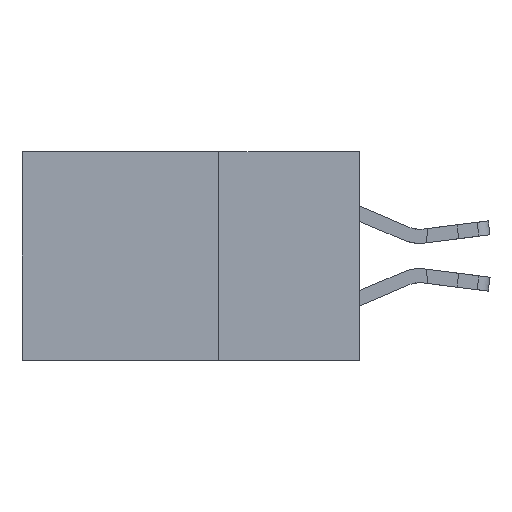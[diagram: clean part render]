
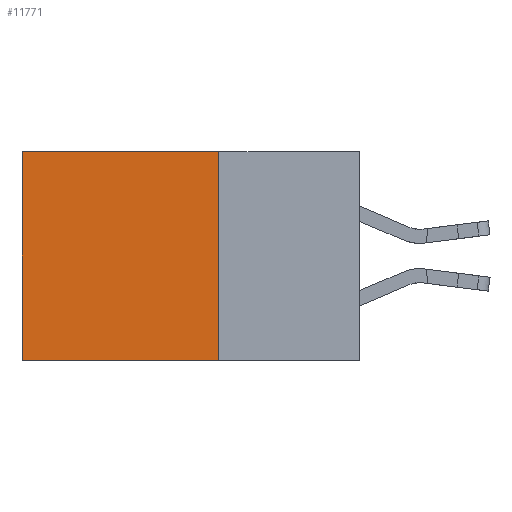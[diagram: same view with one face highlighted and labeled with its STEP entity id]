
A CAD part, left-side view. The second image highlights one B-rep face of the part: STEP entity #11771.
In plain terms, the highlighted planar face has unit normal (-1, 0, 0).
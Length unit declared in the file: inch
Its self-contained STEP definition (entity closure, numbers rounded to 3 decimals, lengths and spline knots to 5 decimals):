
#40 = EDGE_CURVE ( 'NONE', #6525, #1694, #21923, .T. ) ;
#1694 = VERTEX_POINT ( 'NONE', #3701 ) ;
#2074 = VECTOR ( 'NONE', #22208, 39.37008 ) ;
#2262 = CARTESIAN_POINT ( 'NONE',  ( 0.2875, 0.6, -0.37 ) ) ;
#2395 = DIRECTION ( 'NONE',  ( 0., 0., -1. ) ) ;
#2491 = CARTESIAN_POINT ( 'NONE',  ( 0.2875, 0.6, 0. ) ) ;
#3660 = LINE ( 'NONE', #2491, #9148 ) ;
#3701 = CARTESIAN_POINT ( 'NONE',  ( 0.2875, 0.6, 0. ) ) ;
#6525 = VERTEX_POINT ( 'NONE', #13653 ) ;
#6971 = VERTEX_POINT ( 'NONE', #26401 ) ;
#7030 = CARTESIAN_POINT ( 'NONE',  ( 0.2875, 0.25, 0. ) ) ;
#9148 = VECTOR ( 'NONE', #2395, 39.37008 ) ;
#9944 = FACE_OUTER_BOUND ( 'NONE', #11596, .T. ) ;
#10427 = PLANE ( 'NONE',  #12889 ) ;
#10515 = CARTESIAN_POINT ( 'NONE',  ( 0.2875, 0.25, 0. ) ) ;
#10843 = EDGE_CURVE ( 'NONE', #6971, #20252, #19705, .T. ) ;
#11596 = EDGE_LOOP ( 'NONE', ( #14312, #22333, #11752, #15741 ) ) ;
#11752 = ORIENTED_EDGE ( 'NONE', *, *, #15816, .F. ) ;
#11771 = ADVANCED_FACE ( 'NONE', ( #9944 ), #10427, .F. ) ;
#12889 = AXIS2_PLACEMENT_3D ( 'NONE', #10515, #22257, #15390 ) ;
#13653 = CARTESIAN_POINT ( 'NONE',  ( 0.2875, 0.25, 0. ) ) ;
#14096 = EDGE_CURVE ( 'NONE', #1694, #20252, #3660, .T. ) ;
#14312 = ORIENTED_EDGE ( 'NONE', *, *, #14096, .T. ) ;
#14995 = LINE ( 'NONE', #15427, #17056 ) ;
#15390 = DIRECTION ( 'NONE',  ( 0., 0., -1. ) ) ;
#15427 = CARTESIAN_POINT ( 'NONE',  ( 0.2875, 0.25, 0. ) ) ;
#15741 = ORIENTED_EDGE ( 'NONE', *, *, #40, .T. ) ;
#15816 = EDGE_CURVE ( 'NONE', #6525, #6971, #14995, .T. ) ;
#17056 = VECTOR ( 'NONE', #20312, 39.37008 ) ;
#19475 = VECTOR ( 'NONE', #22732, 39.37008 ) ;
#19705 = LINE ( 'NONE', #24545, #2074 ) ;
#20252 = VERTEX_POINT ( 'NONE', #2262 ) ;
#20312 = DIRECTION ( 'NONE',  ( 0., 0., -1. ) ) ;
#21923 = LINE ( 'NONE', #7030, #19475 ) ;
#22208 = DIRECTION ( 'NONE',  ( 0., 1., 0. ) ) ;
#22257 = DIRECTION ( 'NONE',  ( 1., 0., 0. ) ) ;
#22333 = ORIENTED_EDGE ( 'NONE', *, *, #10843, .F. ) ;
#22732 = DIRECTION ( 'NONE',  ( 0., 1., 0. ) ) ;
#24545 = CARTESIAN_POINT ( 'NONE',  ( 0.2875, 0.25, -0.37 ) ) ;
#26401 = CARTESIAN_POINT ( 'NONE',  ( 0.2875, 0.25, -0.37 ) ) ;
